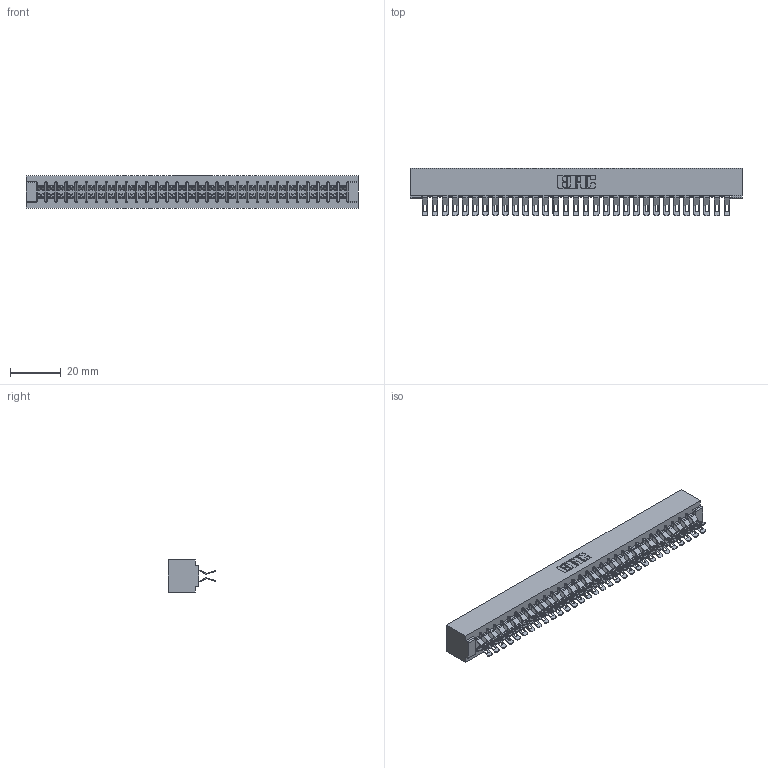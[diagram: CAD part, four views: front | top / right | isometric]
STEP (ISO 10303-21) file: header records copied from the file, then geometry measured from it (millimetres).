
FILE_DESCRIPTION (( 'STEP AP203' ), '1' );
FILE_NAME ('357-062-455-201.STEP', '2020-10-04T15:25:33', ( '' ), ( '' ), 'SwSTEP 2.0', 'SolidWorks 2020', '' );
FILE_SCHEMA (( 'CONFIG_CONTROL_DESIGN' ));
Length unit declared in the file: inch
Products named in the file (3): 307-290-001_555; 307 Part_No Mounting Lugs; 357-062-455-201
Assembly tree (63 placements, depth 2):
  357-062-455-201
    307 Part_No Mounting Lugs
    307-290-001_555  x62
Bounding box: 130.71 x 18.75 x 12.7 mm (x, y, z)
Volume: 14553.6 mm3; surface area: 18925.4 mm2
Topology: 63 solids, 63 shells, 3924 faces, 11521 edges, 7510 vertices
Faces by surface type: plane 2174, cylinder 1686, sphere 64
Entity records: 29183 total; most frequent: CARTESIAN_POINT 4779, ORIENTED_EDGE 4736, DIRECTION 4692, EDGE_CURVE 2368, VECTOR 1802, LINE 1802, VERTEX_POINT 1532, AXIS2_PLACEMENT_3D 1445
